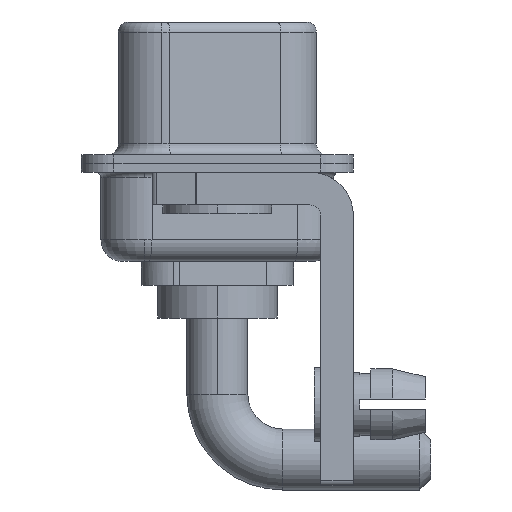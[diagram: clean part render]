
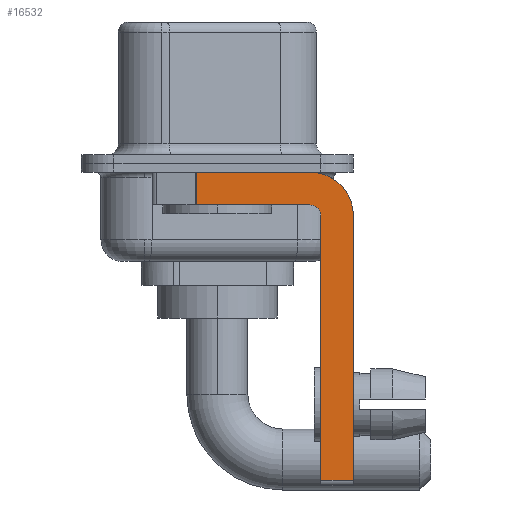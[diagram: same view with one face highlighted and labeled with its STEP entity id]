
A CAD part, left-side view. The second image highlights one B-rep face of the part: STEP entity #16532.
In plain terms, the highlighted planar face has unit normal (-1, 0, 0).
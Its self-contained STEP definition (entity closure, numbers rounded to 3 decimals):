
#412 = DIRECTION ( 'NONE',  ( 0., 0., -1. ) ) ;
#966 = VECTOR ( 'NONE', #14275, 1000. ) ;
#1267 = CARTESIAN_POINT ( 'NONE',  ( -2.9, -4.25, -0.4 ) ) ;
#1516 = VERTEX_POINT ( 'NONE', #2761 ) ;
#1617 = EDGE_CURVE ( 'NONE', #12752, #14108, #3204, .T. ) ;
#1650 = ORIENTED_EDGE ( 'NONE', *, *, #7987, .F. ) ;
#1696 = LINE ( 'NONE', #3229, #13489 ) ;
#2053 = DIRECTION ( 'NONE',  ( 1., 0., 0. ) ) ;
#2153 = DIRECTION ( 'NONE',  ( 0., -1., 0. ) ) ;
#2761 = CARTESIAN_POINT ( 'NONE',  ( -2.9, -6.25, -14.55 ) ) ;
#2813 = CARTESIAN_POINT ( 'NONE',  ( -2.9, -6.25, -2.4 ) ) ;
#3164 = AXIS2_PLACEMENT_3D ( 'NONE', #8936, #7328, #12658 ) ;
#3204 = CIRCLE ( 'NONE', #5115, 2. ) ;
#3229 = CARTESIAN_POINT ( 'NONE',  ( -2.9, 0.978, -1.9 ) ) ;
#3239 = CARTESIAN_POINT ( 'NONE',  ( -2.9, -4.75, -14.55 ) ) ;
#3408 = CARTESIAN_POINT ( 'NONE',  ( -2.9, 0.978, -1.9 ) ) ;
#3772 = PLANE ( 'NONE',  #3164 ) ;
#4023 = DIRECTION ( 'NONE',  ( 0., 0., -1. ) ) ;
#4048 = DIRECTION ( 'NONE',  ( 0., 1., 0. ) ) ;
#4524 = EDGE_CURVE ( 'NONE', #9430, #9072, #9123, .T. ) ;
#4735 = ORIENTED_EDGE ( 'NONE', *, *, #7137, .F. ) ;
#4888 = ORIENTED_EDGE ( 'NONE', *, *, #1617, .F. ) ;
#5115 = AXIS2_PLACEMENT_3D ( 'NONE', #12400, #2053, #13351 ) ;
#5309 = LINE ( 'NONE', #6751, #966 ) ;
#5545 = CARTESIAN_POINT ( 'NONE',  ( -2.9, -6.25, -2.4 ) ) ;
#5617 = VERTEX_POINT ( 'NONE', #3408 ) ;
#5885 = CIRCLE ( 'NONE', #11832, 0.5 ) ;
#6052 = VECTOR ( 'NONE', #4023, 1000. ) ;
#6644 = VERTEX_POINT ( 'NONE', #7352 ) ;
#6751 = CARTESIAN_POINT ( 'NONE',  ( -2.9, -4.25, -14.55 ) ) ;
#6967 = VECTOR ( 'NONE', #2153, 1000. ) ;
#7137 = EDGE_CURVE ( 'NONE', #6644, #5617, #16649, .T. ) ;
#7328 = DIRECTION ( 'NONE',  ( 1., 0., 0. ) ) ;
#7352 = CARTESIAN_POINT ( 'NONE',  ( -2.9, -4.25, -1.9 ) ) ;
#7836 = CARTESIAN_POINT ( 'NONE',  ( -2.9, -4.75, -2.4 ) ) ;
#7915 = ORIENTED_EDGE ( 'NONE', *, *, #12913, .T. ) ;
#7987 = EDGE_CURVE ( 'NONE', #14108, #1516, #10616, .T. ) ;
#8199 = CARTESIAN_POINT ( 'NONE',  ( -2.9, -4.25, -2.4 ) ) ;
#8936 = CARTESIAN_POINT ( 'NONE',  ( -2.9, -4.25, -2.4 ) ) ;
#9072 = VERTEX_POINT ( 'NONE', #7836 ) ;
#9123 = LINE ( 'NONE', #13361, #16021 ) ;
#9430 = VERTEX_POINT ( 'NONE', #3239 ) ;
#10616 = LINE ( 'NONE', #5545, #6052 ) ;
#10725 = DIRECTION ( 'NONE',  ( 0., 0., 1. ) ) ;
#11483 = EDGE_CURVE ( 'NONE', #9072, #6644, #5885, .T. ) ;
#11497 = ORIENTED_EDGE ( 'NONE', *, *, #16514, .F. ) ;
#11832 = AXIS2_PLACEMENT_3D ( 'NONE', #8199, #13441, #10725 ) ;
#12250 = CARTESIAN_POINT ( 'NONE',  ( -2.9, 0.978, -0.4 ) ) ;
#12400 = CARTESIAN_POINT ( 'NONE',  ( -2.9, -4.25, -2.4 ) ) ;
#12658 = DIRECTION ( 'NONE',  ( 0., 0., -1. ) ) ;
#12741 = FACE_OUTER_BOUND ( 'NONE', #13646, .T. ) ;
#12752 = VERTEX_POINT ( 'NONE', #1267 ) ;
#12860 = ORIENTED_EDGE ( 'NONE', *, *, #16618, .T. ) ;
#12913 = EDGE_CURVE ( 'NONE', #16356, #5617, #1696, .T. ) ;
#13274 = DIRECTION ( 'NONE',  ( 0., 0., 1. ) ) ;
#13351 = DIRECTION ( 'NONE',  ( 0., 0., -1. ) ) ;
#13361 = CARTESIAN_POINT ( 'NONE',  ( -2.9, -4.75, -14.8 ) ) ;
#13441 = DIRECTION ( 'NONE',  ( -1., 0., 0. ) ) ;
#13489 = VECTOR ( 'NONE', #412, 1000. ) ;
#13646 = EDGE_LOOP ( 'NONE', ( #11497, #7915, #4735, #14104, #15119, #12860, #1650, #4888 ) ) ;
#13761 = LINE ( 'NONE', #16302, #6967 ) ;
#14104 = ORIENTED_EDGE ( 'NONE', *, *, #11483, .F. ) ;
#14106 = CARTESIAN_POINT ( 'NONE',  ( -2.9, -4.25, -1.9 ) ) ;
#14108 = VERTEX_POINT ( 'NONE', #2813 ) ;
#14275 = DIRECTION ( 'NONE',  ( 0., -1., 0. ) ) ;
#15119 = ORIENTED_EDGE ( 'NONE', *, *, #4524, .F. ) ;
#15812 = VECTOR ( 'NONE', #4048, 1000. ) ;
#16021 = VECTOR ( 'NONE', #13274, 1000. ) ;
#16302 = CARTESIAN_POINT ( 'NONE',  ( -2.9, 3., -0.4 ) ) ;
#16356 = VERTEX_POINT ( 'NONE', #12250 ) ;
#16514 = EDGE_CURVE ( 'NONE', #16356, #12752, #13761, .T. ) ;
#16532 = ADVANCED_FACE ( 'NONE', ( #12741 ), #3772, .F. ) ;
#16618 = EDGE_CURVE ( 'NONE', #9430, #1516, #5309, .T. ) ;
#16649 = LINE ( 'NONE', #14106, #15812 ) ;
